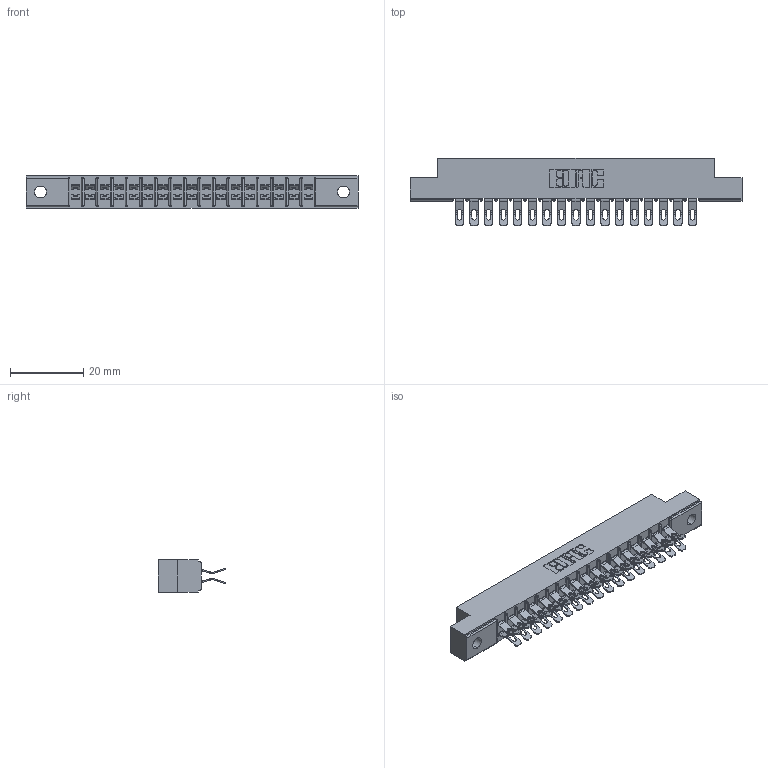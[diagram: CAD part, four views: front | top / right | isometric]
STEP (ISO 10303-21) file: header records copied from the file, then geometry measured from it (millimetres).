
FILE_DESCRIPTION (( 'STEP AP203' ), '1' );
FILE_NAME ('315-034-555-202.STEP', '2019-09-10T15:57:35', ( '' ), ( '' ), 'SwSTEP 2.0', 'SolidWorks 2016', '' );
FILE_SCHEMA (( 'CONFIG_CONTROL_DESIGN' ));
Length unit declared in the file: inch
Products named in the file (3): 305-290-001_555; 305 Part_.128 Dia; 315-034-555-202
Assembly tree (35 placements, depth 2):
  315-034-555-202
    305 Part_.128 Dia
    305-290-001_555  x34
Bounding box: 90.37 x 18.41 x 8.71 mm (x, y, z)
Volume: 5743.3 mm3; surface area: 10865.7 mm2
Topology: 35 solids, 35 shells, 2360 faces, 7031 edges, 4594 vertices
Faces by surface type: plane 1156, cylinder 1136, sphere 68
Entity records: 22076 total; most frequent: CARTESIAN_POINT 3671, ORIENTED_EDGE 3630, DIRECTION 3565, EDGE_CURVE 1815, VECTOR 1421, LINE 1421, VERTEX_POINT 1162, AXIS2_PLACEMENT_3D 1072
